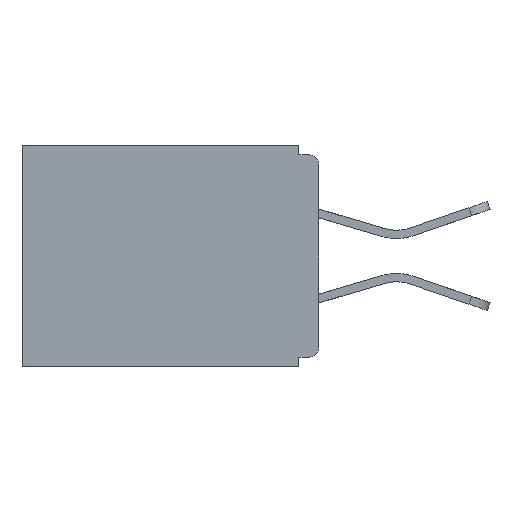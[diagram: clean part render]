
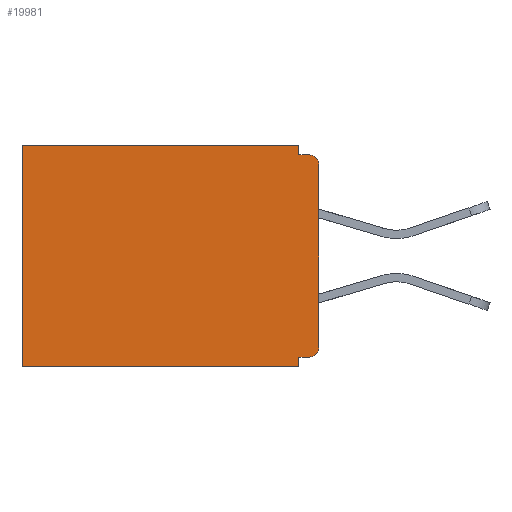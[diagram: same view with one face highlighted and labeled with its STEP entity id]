
A CAD part, left-side view. The second image highlights one B-rep face of the part: STEP entity #19981.
In plain terms, the highlighted planar face has unit normal (-1, 0, 0).
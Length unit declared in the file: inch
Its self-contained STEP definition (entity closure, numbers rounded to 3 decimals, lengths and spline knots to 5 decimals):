
#28 = LINE ( 'NONE', #16496, #18848 ) ;
#364 = DIRECTION ( 'NONE',  ( 0., 1., 0. ) ) ;
#669 = CARTESIAN_POINT ( 'NONE',  ( 0.298, 0.031, -0.328 ) ) ;
#1632 = DIRECTION ( 'NONE',  ( 0., 0., -1. ) ) ;
#1710 = DIRECTION ( 'NONE',  ( 0., 0., -1. ) ) ;
#1950 = VERTEX_POINT ( 'NONE', #14226 ) ;
#2073 = LINE ( 'NONE', #23277, #5428 ) ;
#2200 = ORIENTED_EDGE ( 'NONE', *, *, #14255, .T. ) ;
#2288 = EDGE_CURVE ( 'NONE', #25534, #3002, #28, .T. ) ;
#2560 = CARTESIAN_POINT ( 'NONE',  ( 0.298, 0.015, -0.313 ) ) ;
#3002 = VERTEX_POINT ( 'NONE', #19042 ) ;
#3091 = CARTESIAN_POINT ( 'NONE',  ( 0.298, 0., -0.343 ) ) ;
#3498 = DIRECTION ( 'NONE',  ( 0., 0., -1. ) ) ;
#3596 = VECTOR ( 'NONE', #22236, 39.37008 ) ;
#3692 = VERTEX_POINT ( 'NONE', #669 ) ;
#3805 = VECTOR ( 'NONE', #1710, 39.37008 ) ;
#4066 = ORIENTED_EDGE ( 'NONE', *, *, #14853, .F. ) ;
#4431 = DIRECTION ( 'NONE',  ( 0., 1., 0. ) ) ;
#5294 = LINE ( 'NONE', #18433, #6828 ) ;
#5393 = DIRECTION ( 'NONE',  ( 0., 1., 0. ) ) ;
#5428 = VECTOR ( 'NONE', #15054, 39.37008 ) ;
#5458 = CARTESIAN_POINT ( 'NONE',  ( 0.298, 0.015, -0.03 ) ) ;
#5806 = ORIENTED_EDGE ( 'NONE', *, *, #17909, .T. ) ;
#5855 = CARTESIAN_POINT ( 'NONE',  ( 0.298, 0., 0. ) ) ;
#6039 = VERTEX_POINT ( 'NONE', #21756 ) ;
#6275 = DIRECTION ( 'NONE',  ( 0., 0., -1. ) ) ;
#6472 = CARTESIAN_POINT ( 'NONE',  ( 0.298, 0., -0.015 ) ) ;
#6579 = CARTESIAN_POINT ( 'NONE',  ( 0.298, 0., -0.03 ) ) ;
#6828 = VECTOR ( 'NONE', #364, 39.37008 ) ;
#6922 = ORIENTED_EDGE ( 'NONE', *, *, #17127, .F. ) ;
#7441 = CARTESIAN_POINT ( 'NONE',  ( 0.298, 0.46, 0. ) ) ;
#8422 = DIRECTION ( 'NONE',  ( -1., 0., 0. ) ) ;
#9084 = VECTOR ( 'NONE', #5393, 39.37008 ) ;
#9088 = ORIENTED_EDGE ( 'NONE', *, *, #18831, .T. ) ;
#9204 = CARTESIAN_POINT ( 'NONE',  ( 0.298, 0., 0. ) ) ;
#9383 = DIRECTION ( 'NONE',  ( 0., 0., -1. ) ) ;
#9398 = CARTESIAN_POINT ( 'NONE',  ( 0.298, 0.031, -0.343 ) ) ;
#9718 = EDGE_CURVE ( 'NONE', #11592, #6039, #16361, .T. ) ;
#9841 = FACE_OUTER_BOUND ( 'NONE', #23723, .T. ) ;
#10175 = CIRCLE ( 'NONE', #14908, 0.015 ) ;
#10521 = LINE ( 'NONE', #18177, #11151 ) ;
#11038 = DIRECTION ( 'NONE',  ( 1., 0., 0. ) ) ;
#11151 = VECTOR ( 'NONE', #4431, 39.37008 ) ;
#11197 = DIRECTION ( 'NONE',  ( -1., 0., 0. ) ) ;
#11386 = ORIENTED_EDGE ( 'NONE', *, *, #12983, .F. ) ;
#11549 = CARTESIAN_POINT ( 'NONE',  ( 0.298, 0.015, -0.328 ) ) ;
#11592 = VERTEX_POINT ( 'NONE', #6579 ) ;
#11890 = EDGE_CURVE ( 'NONE', #14578, #22918, #18120, .T. ) ;
#12090 = ORIENTED_EDGE ( 'NONE', *, *, #11890, .F. ) ;
#12599 = AXIS2_PLACEMENT_3D ( 'NONE', #9204, #11038, #9383 ) ;
#12799 = ORIENTED_EDGE ( 'NONE', *, *, #15087, .F. ) ;
#12983 = EDGE_CURVE ( 'NONE', #20268, #3002, #14352, .T. ) ;
#13862 = AXIS2_PLACEMENT_3D ( 'NONE', #5458, #11197, #3498 ) ;
#14226 = CARTESIAN_POINT ( 'NONE',  ( 0.298, 0.031, 0. ) ) ;
#14255 = EDGE_CURVE ( 'NONE', #11592, #22918, #18925, .T. ) ;
#14352 = LINE ( 'NONE', #3091, #9084 ) ;
#14578 = VERTEX_POINT ( 'NONE', #21582 ) ;
#14837 = VECTOR ( 'NONE', #1632, 39.37008 ) ;
#14853 = EDGE_CURVE ( 'NONE', #18349, #3692, #5294, .T. ) ;
#14908 = AXIS2_PLACEMENT_3D ( 'NONE', #2560, #8422, #20360 ) ;
#15054 = DIRECTION ( 'NONE',  ( 0., 0., -1. ) ) ;
#15087 = EDGE_CURVE ( 'NONE', #1950, #14578, #2073, .T. ) ;
#16361 = LINE ( 'NONE', #5855, #14837 ) ;
#16496 = CARTESIAN_POINT ( 'NONE',  ( 0.298, 0.46, 0. ) ) ;
#17127 = EDGE_CURVE ( 'NONE', #3692, #20268, #19583, .T. ) ;
#17909 = EDGE_CURVE ( 'NONE', #1950, #25534, #10521, .T. ) ;
#18120 = LINE ( 'NONE', #6472, #3596 ) ;
#18177 = CARTESIAN_POINT ( 'NONE',  ( 0.298, 0., 0. ) ) ;
#18349 = VERTEX_POINT ( 'NONE', #11549 ) ;
#18433 = CARTESIAN_POINT ( 'NONE',  ( 0.298, 0., -0.328 ) ) ;
#18831 = EDGE_CURVE ( 'NONE', #18349, #6039, #10175, .T. ) ;
#18848 = VECTOR ( 'NONE', #6275, 39.37008 ) ;
#18925 = CIRCLE ( 'NONE', #13862, 0.015 ) ;
#19042 = CARTESIAN_POINT ( 'NONE',  ( 0.298, 0.46, -0.343 ) ) ;
#19583 = LINE ( 'NONE', #9398, #3805 ) ;
#19981 = ADVANCED_FACE ( 'NONE', ( #9841 ), #20988, .F. ) ;
#20268 = VERTEX_POINT ( 'NONE', #24108 ) ;
#20360 = DIRECTION ( 'NONE',  ( 0., 0., -1. ) ) ;
#20988 = PLANE ( 'NONE',  #12599 ) ;
#21582 = CARTESIAN_POINT ( 'NONE',  ( 0.298, 0.031, -0.015 ) ) ;
#21756 = CARTESIAN_POINT ( 'NONE',  ( 0.298, 0., -0.313 ) ) ;
#22236 = DIRECTION ( 'NONE',  ( 0., -1., 0. ) ) ;
#22581 = ORIENTED_EDGE ( 'NONE', *, *, #9718, .F. ) ;
#22918 = VERTEX_POINT ( 'NONE', #25281 ) ;
#23277 = CARTESIAN_POINT ( 'NONE',  ( 0.298, 0.031, -0.343 ) ) ;
#23723 = EDGE_LOOP ( 'NONE', ( #2200, #12090, #12799, #5806, #23877, #11386, #6922, #4066, #9088, #22581 ) ) ;
#23877 = ORIENTED_EDGE ( 'NONE', *, *, #2288, .T. ) ;
#24108 = CARTESIAN_POINT ( 'NONE',  ( 0.298, 0.031, -0.343 ) ) ;
#25281 = CARTESIAN_POINT ( 'NONE',  ( 0.298, 0.015, -0.015 ) ) ;
#25534 = VERTEX_POINT ( 'NONE', #7441 ) ;
